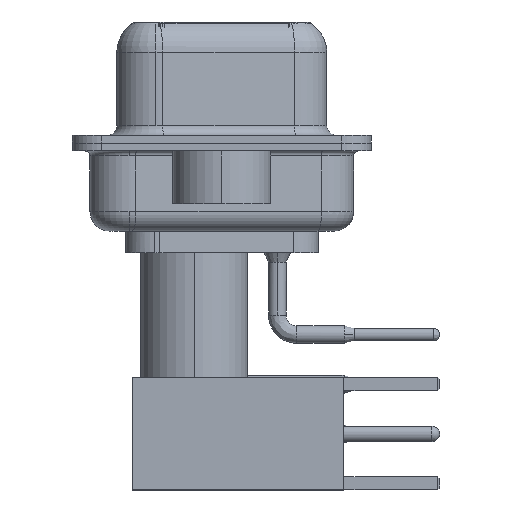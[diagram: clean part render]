
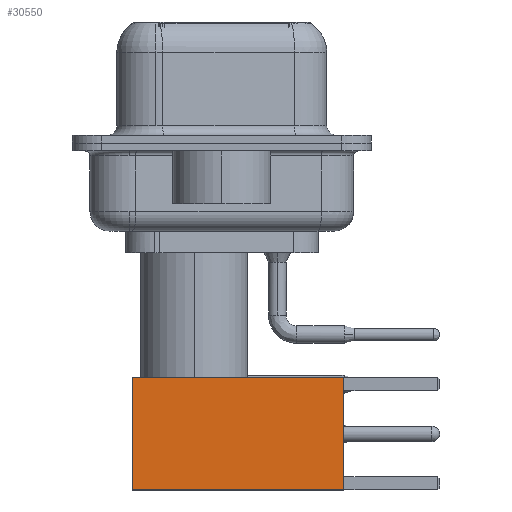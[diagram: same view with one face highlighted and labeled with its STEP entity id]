
A CAD part, left-side view. The second image highlights one B-rep face of the part: STEP entity #30550.
In plain terms, the highlighted face is planar.
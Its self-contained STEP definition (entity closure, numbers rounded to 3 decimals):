
#161 = DIRECTION ( 'NONE',  ( -1., 0., 0. ) ) ;
#349 = VECTOR ( 'NONE', #17359, 1000. ) ;
#1071 = LINE ( 'NONE', #33238, #1605 ) ;
#1605 = VECTOR ( 'NONE', #161, 1000. ) ;
#1865 = LINE ( 'NONE', #27136, #349 ) ;
#2001 = ORIENTED_EDGE ( 'NONE', *, *, #6547, .T. ) ;
#2304 = VERTEX_POINT ( 'NONE', #21102 ) ;
#2885 = ORIENTED_EDGE ( 'NONE', *, *, #31160, .F. ) ;
#2958 = VERTEX_POINT ( 'NONE', #14619 ) ;
#3317 = CARTESIAN_POINT ( 'NONE',  ( 2.875, 2.875, 0. ) ) ;
#3634 = FACE_OUTER_BOUND ( 'NONE', #25514, .T. ) ;
#4065 = VERTEX_POINT ( 'NONE', #12350 ) ;
#6547 = EDGE_CURVE ( 'NONE', #2958, #2304, #1865, .T. ) ;
#7455 = LINE ( 'NONE', #17734, #26111 ) ;
#8031 = PLANE ( 'NONE',  #29599 ) ;
#9627 = CARTESIAN_POINT ( 'NONE',  ( 2.875, 2.875, 10.82 ) ) ;
#10302 = ORIENTED_EDGE ( 'NONE', *, *, #17930, .F. ) ;
#11492 = CARTESIAN_POINT ( 'NONE',  ( 2.875, 2.875, 0. ) ) ;
#12350 = CARTESIAN_POINT ( 'NONE',  ( -2.875, 2.875, 10.82 ) ) ;
#14619 = CARTESIAN_POINT ( 'NONE',  ( 2.875, 2.875, 0. ) ) ;
#16584 = VECTOR ( 'NONE', #17032, 1000. ) ;
#17032 = DIRECTION ( 'NONE',  ( 0., 0., -1. ) ) ;
#17359 = DIRECTION ( 'NONE',  ( -1., 0., 0. ) ) ;
#17734 = CARTESIAN_POINT ( 'NONE',  ( -2.875, 2.875, 0. ) ) ;
#17930 = EDGE_CURVE ( 'NONE', #4065, #2304, #7455, .T. ) ;
#19612 = DIRECTION ( 'NONE',  ( 0., 0., -1. ) ) ;
#21102 = CARTESIAN_POINT ( 'NONE',  ( -2.875, 2.875, 0. ) ) ;
#22165 = ORIENTED_EDGE ( 'NONE', *, *, #22631, .T. ) ;
#22631 = EDGE_CURVE ( 'NONE', #32997, #2958, #32588, .T. ) ;
#25514 = EDGE_LOOP ( 'NONE', ( #22165, #2001, #10302, #2885 ) ) ;
#26111 = VECTOR ( 'NONE', #19612, 1000. ) ;
#27136 = CARTESIAN_POINT ( 'NONE',  ( 0., 2.875, 0. ) ) ;
#28604 = DIRECTION ( 'NONE',  ( 0., 1., 0. ) ) ;
#29109 = DIRECTION ( 'NONE',  ( 0., 0., 1. ) ) ;
#29599 = AXIS2_PLACEMENT_3D ( 'NONE', #3317, #28604, #29109 ) ;
#30550 = ADVANCED_FACE ( 'NONE', ( #3634 ), #8031, .T. ) ;
#31160 = EDGE_CURVE ( 'NONE', #32997, #4065, #1071, .T. ) ;
#32588 = LINE ( 'NONE', #11492, #16584 ) ;
#32997 = VERTEX_POINT ( 'NONE', #9627 ) ;
#33238 = CARTESIAN_POINT ( 'NONE',  ( 0., 2.875, 10.82 ) ) ;
